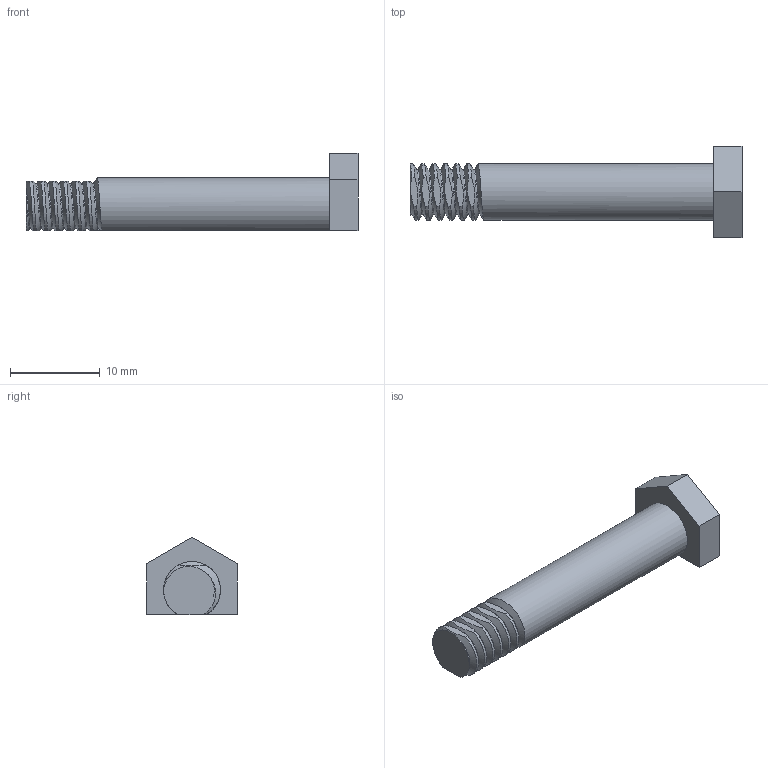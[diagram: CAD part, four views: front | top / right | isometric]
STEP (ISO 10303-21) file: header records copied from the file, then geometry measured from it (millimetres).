
FILE_DESCRIPTION (( 'STEP AP203' ), '1' );
FILE_NAME ('AF-WF-GS-PRT-003-STEP.STEP', '2020-07-21T18:59:52', ( '' ), ( '' ), 'SwSTEP 2.0', 'SolidWorks 2018', '' );
FILE_SCHEMA (( 'CONFIG_CONTROL_DESIGN' ));
Length unit declared in the file: inch
Products named in the file (1): AF-WF-GS-PRT-003-STEP
Bounding box: 37.08 x 10.16 x 8.61 mm (x, y, z)
Volume: 1230 mm3; surface area: 978.8 mm2
Topology: 1 solids, 1 shells, 37 faces, 105 edges, 70 vertices
Faces by surface type: plane 21, cylinder 13, bspline 3
Entity records: 2415 total; most frequent: CARTESIAN_POINT 1519, ORIENTED_EDGE 210, DIRECTION 121, EDGE_CURVE 105, VERTEX_POINT 70, VECTOR 47, LINE 47, ADVANCED_FACE 37
